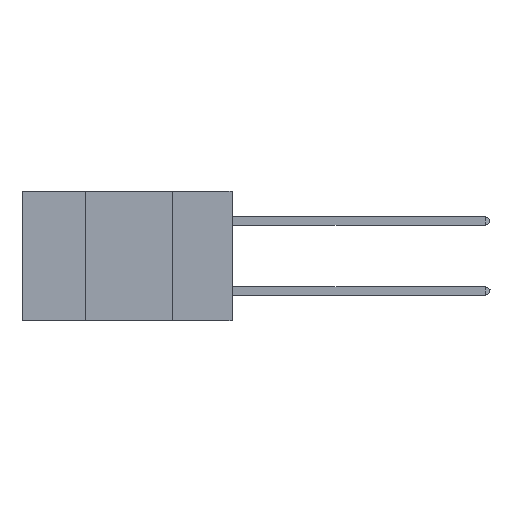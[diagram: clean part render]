
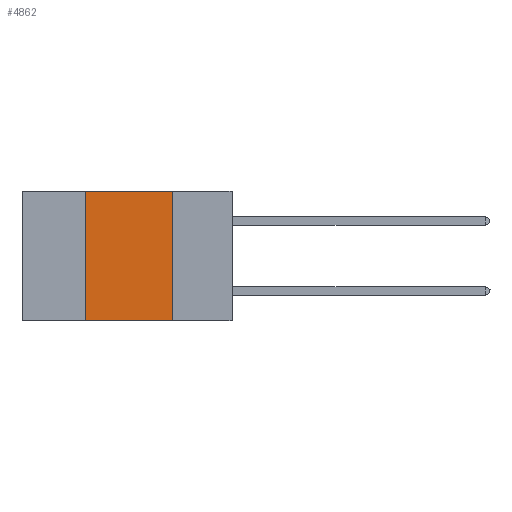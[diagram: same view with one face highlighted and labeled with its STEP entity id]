
A CAD part, left-side view. The second image highlights one B-rep face of the part: STEP entity #4862.
In plain terms, the highlighted planar face has unit normal (-1, 0, 0).
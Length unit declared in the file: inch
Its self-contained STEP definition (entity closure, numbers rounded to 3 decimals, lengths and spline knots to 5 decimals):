
#171 = EDGE_CURVE ( 'NONE', #9951, #799, #34332, .T. ) ;
#799 = VERTEX_POINT ( 'NONE', #9517 ) ;
#4224 = CARTESIAN_POINT ( 'NONE',  ( 0., 0.17, 0. ) ) ;
#4699 = DIRECTION ( 'NONE',  ( 0., 0., 1. ) ) ;
#4862 = ADVANCED_FACE ( 'NONE', ( #29222 ), #36193, .F. ) ;
#4898 = EDGE_CURVE ( 'NONE', #23652, #799, #46395, .T. ) ;
#6811 = DIRECTION ( 'NONE',  ( 0., 0., -1. ) ) ;
#8334 = EDGE_LOOP ( 'NONE', ( #14066, #27346, #24472, #26792 ) ) ;
#8918 = AXIS2_PLACEMENT_3D ( 'NONE', #10388, #14101, #39870 ) ;
#9517 = CARTESIAN_POINT ( 'NONE',  ( 0., 0.17, -0.37 ) ) ;
#9951 = VERTEX_POINT ( 'NONE', #29049 ) ;
#10388 = CARTESIAN_POINT ( 'NONE',  ( 0., 0.6, 0. ) ) ;
#13906 = EDGE_CURVE ( 'NONE', #41875, #23652, #42386, .T. ) ;
#14066 = ORIENTED_EDGE ( 'NONE', *, *, #4898, .F. ) ;
#14101 = DIRECTION ( 'NONE',  ( 1., 0., 0. ) ) ;
#14201 = VECTOR ( 'NONE', #36265, 39.37008 ) ;
#17163 = DIRECTION ( 'NONE',  ( 0., -1., 0. ) ) ;
#21764 = EDGE_CURVE ( 'NONE', #9951, #41875, #43077, .T. ) ;
#23652 = VERTEX_POINT ( 'NONE', #4224 ) ;
#24068 = CARTESIAN_POINT ( 'NONE',  ( 0., 0.42, 0. ) ) ;
#24472 = ORIENTED_EDGE ( 'NONE', *, *, #21764, .F. ) ;
#26792 = ORIENTED_EDGE ( 'NONE', *, *, #171, .T. ) ;
#27346 = ORIENTED_EDGE ( 'NONE', *, *, #13906, .F. ) ;
#28851 = CARTESIAN_POINT ( 'NONE',  ( 0., 0.6, 0. ) ) ;
#29049 = CARTESIAN_POINT ( 'NONE',  ( 0., 0.42, -0.37 ) ) ;
#29222 = FACE_OUTER_BOUND ( 'NONE', #8334, .T. ) ;
#30367 = CARTESIAN_POINT ( 'NONE',  ( 0., 0.42, 0. ) ) ;
#33182 = VECTOR ( 'NONE', #17163, 39.37008 ) ;
#33357 = VECTOR ( 'NONE', #4699, 39.37008 ) ;
#34332 = LINE ( 'NONE', #39236, #33182 ) ;
#36193 = PLANE ( 'NONE',  #8918 ) ;
#36265 = DIRECTION ( 'NONE',  ( 0., -1., 0. ) ) ;
#36721 = VECTOR ( 'NONE', #6811, 39.37008 ) ;
#39236 = CARTESIAN_POINT ( 'NONE',  ( 0., 0.6, -0.37 ) ) ;
#39870 = DIRECTION ( 'NONE',  ( 0., 0., -1. ) ) ;
#41875 = VERTEX_POINT ( 'NONE', #24068 ) ;
#42386 = LINE ( 'NONE', #28851, #14201 ) ;
#43077 = LINE ( 'NONE', #30367, #33357 ) ;
#46395 = LINE ( 'NONE', #47191, #36721 ) ;
#47191 = CARTESIAN_POINT ( 'NONE',  ( 0., 0.17, 0. ) ) ;
